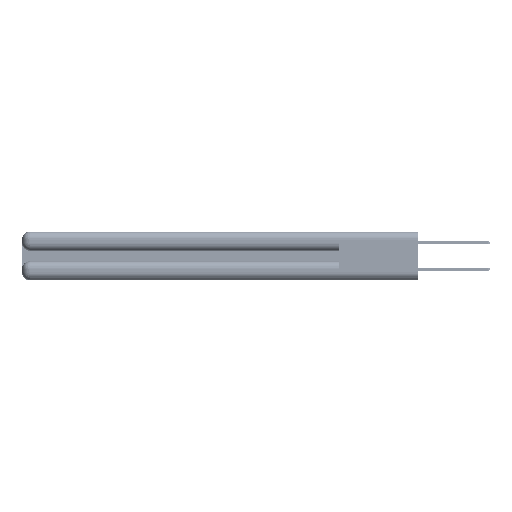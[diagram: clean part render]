
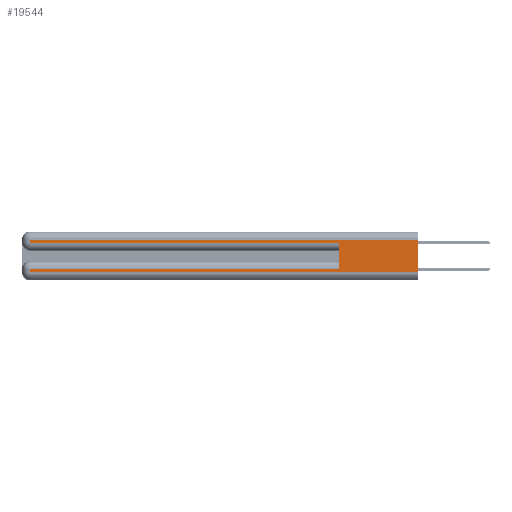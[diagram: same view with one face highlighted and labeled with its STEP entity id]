
A CAD part, left-side view. The second image highlights one B-rep face of the part: STEP entity #19544.
In plain terms, the highlighted planar face has unit normal (-1, 0, 0).
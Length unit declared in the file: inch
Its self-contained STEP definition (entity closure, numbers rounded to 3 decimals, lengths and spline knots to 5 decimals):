
#301 = EDGE_CURVE ( 'NONE', #21980, #30576, #1628, .T. ) ;
#397 = CARTESIAN_POINT ( 'NONE',  ( 0., 0., 0.085 ) ) ;
#1628 = LINE ( 'NONE', #13360, #44483 ) ;
#2193 = CARTESIAN_POINT ( 'NONE',  ( 0., 2.94, 0.06 ) ) ;
#2892 = CARTESIAN_POINT ( 'NONE',  ( 0., 0., 0.37 ) ) ;
#3202 = ORIENTED_EDGE ( 'NONE', *, *, #15155, .T. ) ;
#4009 = CARTESIAN_POINT ( 'NONE',  ( 0., 2.94, 0.37 ) ) ;
#4098 = ORIENTED_EDGE ( 'NONE', *, *, #36126, .T. ) ;
#4982 = LINE ( 'NONE', #15935, #12140 ) ;
#5387 = CARTESIAN_POINT ( 'NONE',  ( 0., 0.6, 0.085 ) ) ;
#6646 = DIRECTION ( 'NONE',  ( 0., 1., 0. ) ) ;
#6793 = CARTESIAN_POINT ( 'NONE',  ( 0., 0.6, 0.285 ) ) ;
#6981 = EDGE_CURVE ( 'NONE', #33377, #51620, #11520, .T. ) ;
#7853 = VECTOR ( 'NONE', #41969, 39.37008 ) ;
#8651 = LINE ( 'NONE', #31682, #28110 ) ;
#11520 = LINE ( 'NONE', #25717, #41958 ) ;
#11669 = CARTESIAN_POINT ( 'NONE',  ( 0., 0., 0.285 ) ) ;
#12140 = VECTOR ( 'NONE', #20114, 39.37008 ) ;
#12633 = EDGE_CURVE ( 'NONE', #20938, #39086, #34340, .T. ) ;
#13216 = DIRECTION ( 'NONE',  ( 0., 0., -1. ) ) ;
#13360 = CARTESIAN_POINT ( 'NONE',  ( 0., 2.94, 0.37 ) ) ;
#15155 = EDGE_CURVE ( 'NONE', #30576, #39086, #34139, .T. ) ;
#15935 = CARTESIAN_POINT ( 'NONE',  ( 0., 0., 0.06 ) ) ;
#15963 = AXIS2_PLACEMENT_3D ( 'NONE', #2892, #19608, #48590 ) ;
#16351 = DIRECTION ( 'NONE',  ( 0., 0., 1. ) ) ;
#19544 = ADVANCED_FACE ( 'NONE', ( #31494 ), #44428, .F. ) ;
#19608 = DIRECTION ( 'NONE',  ( 1., 0., 0. ) ) ;
#20080 = CARTESIAN_POINT ( 'NONE',  ( 0., 0., 0.06 ) ) ;
#20114 = DIRECTION ( 'NONE',  ( 0., -1., 0. ) ) ;
#20182 = LINE ( 'NONE', #397, #7853 ) ;
#20938 = VERTEX_POINT ( 'NONE', #5387 ) ;
#21678 = DIRECTION ( 'NONE',  ( 0., 0., -1. ) ) ;
#21980 = VERTEX_POINT ( 'NONE', #45139 ) ;
#23082 = VECTOR ( 'NONE', #48957, 39.37008 ) ;
#23348 = EDGE_CURVE ( 'NONE', #45820, #43528, #25880, .T. ) ;
#24585 = VECTOR ( 'NONE', #45565, 39.37008 ) ;
#24725 = CARTESIAN_POINT ( 'NONE',  ( 0., 0.6, 0.145 ) ) ;
#24865 = CARTESIAN_POINT ( 'NONE',  ( 0., 2.94, 0.085 ) ) ;
#25717 = CARTESIAN_POINT ( 'NONE',  ( 0., 0., 0.37 ) ) ;
#25880 = LINE ( 'NONE', #4009, #24585 ) ;
#26795 = ORIENTED_EDGE ( 'NONE', *, *, #12633, .F. ) ;
#28110 = VECTOR ( 'NONE', #6646, 39.37008 ) ;
#30576 = VERTEX_POINT ( 'NONE', #42158 ) ;
#31494 = FACE_OUTER_BOUND ( 'NONE', #31541, .T. ) ;
#31541 = EDGE_LOOP ( 'NONE', ( #35652, #41474, #40160, #3202, #26795, #39341, #50130, #4098 ) ) ;
#31682 = CARTESIAN_POINT ( 'NONE',  ( 0., 0., 0.31 ) ) ;
#33377 = VERTEX_POINT ( 'NONE', #41504 ) ;
#34139 = LINE ( 'NONE', #11669, #23082 ) ;
#34340 = LINE ( 'NONE', #24725, #44012 ) ;
#35652 = ORIENTED_EDGE ( 'NONE', *, *, #6981, .F. ) ;
#36126 = EDGE_CURVE ( 'NONE', #43528, #51620, #4982, .T. ) ;
#39086 = VERTEX_POINT ( 'NONE', #6793 ) ;
#39341 = ORIENTED_EDGE ( 'NONE', *, *, #44502, .T. ) ;
#40160 = ORIENTED_EDGE ( 'NONE', *, *, #301, .T. ) ;
#41474 = ORIENTED_EDGE ( 'NONE', *, *, #48337, .T. ) ;
#41504 = CARTESIAN_POINT ( 'NONE',  ( 0., 0., 0.31 ) ) ;
#41958 = VECTOR ( 'NONE', #13216, 39.37008 ) ;
#41969 = DIRECTION ( 'NONE',  ( 0., 1., 0. ) ) ;
#42158 = CARTESIAN_POINT ( 'NONE',  ( 0., 2.94, 0.285 ) ) ;
#43528 = VERTEX_POINT ( 'NONE', #2193 ) ;
#44012 = VECTOR ( 'NONE', #16351, 39.37008 ) ;
#44428 = PLANE ( 'NONE',  #15963 ) ;
#44483 = VECTOR ( 'NONE', #21678, 39.37008 ) ;
#44502 = EDGE_CURVE ( 'NONE', #20938, #45820, #20182, .T. ) ;
#45139 = CARTESIAN_POINT ( 'NONE',  ( 0., 2.94, 0.31 ) ) ;
#45565 = DIRECTION ( 'NONE',  ( 0., 0., -1. ) ) ;
#45820 = VERTEX_POINT ( 'NONE', #24865 ) ;
#48337 = EDGE_CURVE ( 'NONE', #33377, #21980, #8651, .T. ) ;
#48590 = DIRECTION ( 'NONE',  ( 0., 0., -1. ) ) ;
#48957 = DIRECTION ( 'NONE',  ( 0., -1., 0. ) ) ;
#50130 = ORIENTED_EDGE ( 'NONE', *, *, #23348, .T. ) ;
#51620 = VERTEX_POINT ( 'NONE', #20080 ) ;
